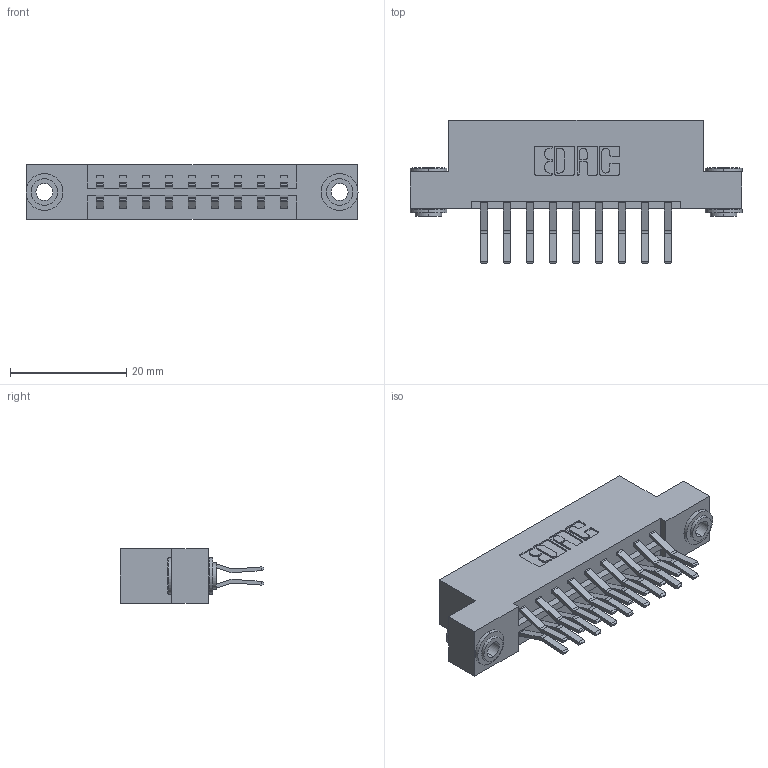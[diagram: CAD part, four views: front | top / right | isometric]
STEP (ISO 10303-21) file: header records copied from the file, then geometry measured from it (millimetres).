
FILE_DESCRIPTION (( 'STEP AP203' ), '1' );
FILE_NAME ('333-018-560-203.STEP', '2019-08-09T14:29:06', ( '' ), ( '' ), 'SwSTEP 2.0', 'SolidWorks 2016', '' );
FILE_SCHEMA (( 'CONFIG_CONTROL_DESIGN' ));
Length unit declared in the file: inch
Products named in the file (4): 345-250-002_345-250-002-102; 333-018-560-203; 345-292-001_560 Tail; 333 Part_Flush - .156 Dia - TH
Assembly tree (21 placements, depth 2):
  333-018-560-203
    333 Part_Flush - .156 Dia - TH
    345-292-001_560 Tail  x18
    345-250-002_345-250-002-102  x2
Bounding box: 57.2 x 24.78 x 9.4 mm (x, y, z)
Volume: 5668.6 mm3; surface area: 6904.6 mm2
Topology: 21 solids, 21 shells, 1124 faces, 3285 edges, 2162 vertices
Faces by surface type: plane 728, cylinder 388, cone 8
Entity records: 10796 total; most frequent: CARTESIAN_POINT 1805, ORIENTED_EDGE 1734, DIRECTION 1637, EDGE_CURVE 867, LINE 711, VECTOR 711, VERTEX_POINT 574, AXIS2_PLACEMENT_3D 463
